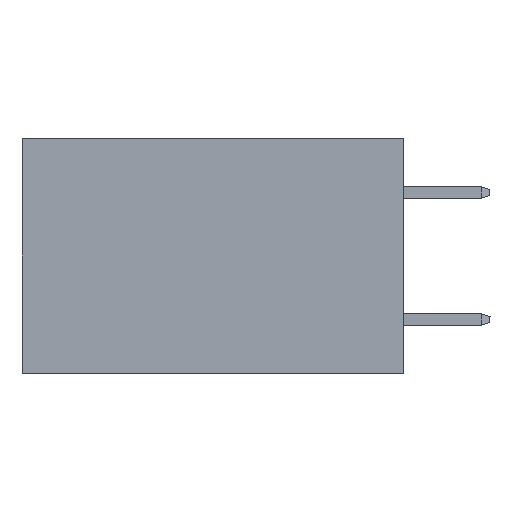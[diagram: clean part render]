
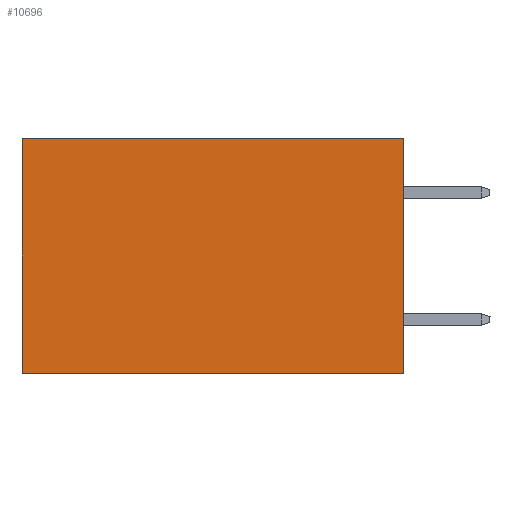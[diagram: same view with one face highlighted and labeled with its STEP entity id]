
A CAD part, left-side view. The second image highlights one B-rep face of the part: STEP entity #10696.
In plain terms, the highlighted planar face has unit normal (-1, 0, 0).
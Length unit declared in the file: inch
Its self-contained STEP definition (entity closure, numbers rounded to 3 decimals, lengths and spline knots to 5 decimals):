
#436 = EDGE_CURVE ( 'NONE', #11839, #2895, #5151, .T. ) ;
#458 = PLANE ( 'NONE',  #9454 ) ;
#854 = VECTOR ( 'NONE', #10844, 39.37008 ) ;
#1598 = DIRECTION ( 'NONE',  ( 0., 1., 0. ) ) ;
#1655 = EDGE_CURVE ( 'NONE', #11839, #9215, #9607, .T. ) ;
#2377 = VECTOR ( 'NONE', #9728, 39.37008 ) ;
#2895 = VERTEX_POINT ( 'NONE', #4665 ) ;
#3846 = LINE ( 'NONE', #8716, #2377 ) ;
#3848 = CARTESIAN_POINT ( 'NONE',  ( 0.2875, 0., 0. ) ) ;
#3911 = CARTESIAN_POINT ( 'NONE',  ( 0.2875, 0., 0. ) ) ;
#4526 = VECTOR ( 'NONE', #1598, 39.37008 ) ;
#4665 = CARTESIAN_POINT ( 'NONE',  ( 0.2875, 0.6, 0. ) ) ;
#4788 = CARTESIAN_POINT ( 'NONE',  ( 0.2875, 0., -0.37 ) ) ;
#5151 = LINE ( 'NONE', #3911, #4526 ) ;
#7649 = FACE_OUTER_BOUND ( 'NONE', #9154, .T. ) ;
#8428 = CARTESIAN_POINT ( 'NONE',  ( 0.2875, 0., 0. ) ) ;
#8571 = VECTOR ( 'NONE', #11283, 39.37008 ) ;
#8716 = CARTESIAN_POINT ( 'NONE',  ( 0.2875, 0., -0.37 ) ) ;
#8717 = DIRECTION ( 'NONE',  ( 0., 0., -1. ) ) ;
#9154 = EDGE_LOOP ( 'NONE', ( #10523, #9918, #13629, #14865 ) ) ;
#9215 = VERTEX_POINT ( 'NONE', #4788 ) ;
#9445 = EDGE_CURVE ( 'NONE', #9215, #9684, #3846, .T. ) ;
#9454 = AXIS2_PLACEMENT_3D ( 'NONE', #3848, #13568, #8717 ) ;
#9607 = LINE ( 'NONE', #14285, #854 ) ;
#9684 = VERTEX_POINT ( 'NONE', #10857 ) ;
#9728 = DIRECTION ( 'NONE',  ( 0., 1., 0. ) ) ;
#9918 = ORIENTED_EDGE ( 'NONE', *, *, #9445, .F. ) ;
#10523 = ORIENTED_EDGE ( 'NONE', *, *, #14566, .T. ) ;
#10696 = ADVANCED_FACE ( 'NONE', ( #7649 ), #458, .F. ) ;
#10844 = DIRECTION ( 'NONE',  ( 0., 0., -1. ) ) ;
#10857 = CARTESIAN_POINT ( 'NONE',  ( 0.2875, 0.6, -0.37 ) ) ;
#11283 = DIRECTION ( 'NONE',  ( 0., 0., -1. ) ) ;
#11839 = VERTEX_POINT ( 'NONE', #8428 ) ;
#13079 = CARTESIAN_POINT ( 'NONE',  ( 0.2875, 0.6, 0. ) ) ;
#13568 = DIRECTION ( 'NONE',  ( 1., 0., 0. ) ) ;
#13589 = LINE ( 'NONE', #13079, #8571 ) ;
#13629 = ORIENTED_EDGE ( 'NONE', *, *, #1655, .F. ) ;
#14285 = CARTESIAN_POINT ( 'NONE',  ( 0.2875, 0., 0. ) ) ;
#14566 = EDGE_CURVE ( 'NONE', #2895, #9684, #13589, .T. ) ;
#14865 = ORIENTED_EDGE ( 'NONE', *, *, #436, .T. ) ;
